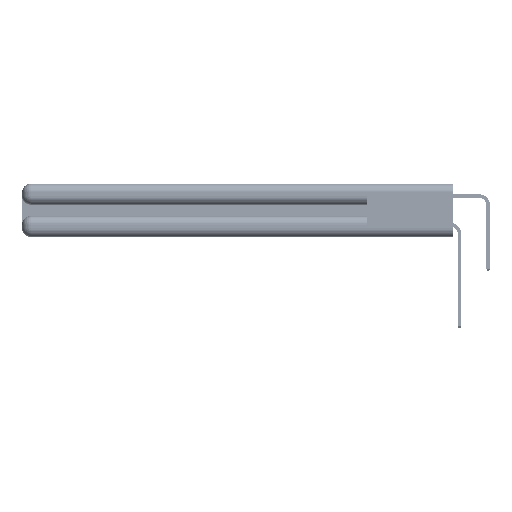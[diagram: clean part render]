
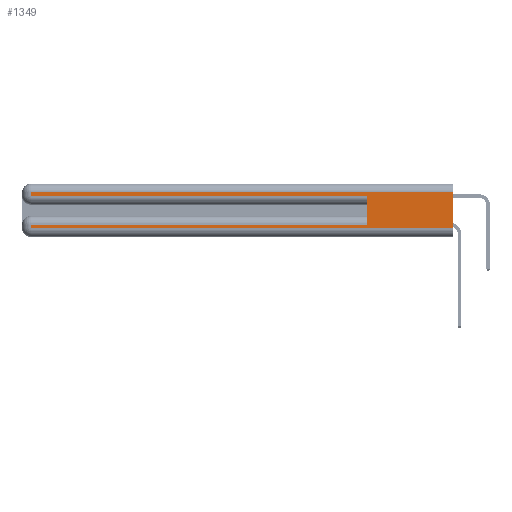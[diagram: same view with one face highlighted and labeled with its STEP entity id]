
A CAD part, left-side view. The second image highlights one B-rep face of the part: STEP entity #1349.
In plain terms, the highlighted planar face has unit normal (-1, 0, 0).
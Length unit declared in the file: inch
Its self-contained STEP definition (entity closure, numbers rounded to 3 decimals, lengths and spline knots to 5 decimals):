
#1305 = VERTEX_POINT ( 'NONE', #24181 ) ;
#1349 = ADVANCED_FACE ( 'NONE', ( #40857 ), #50335, .F. ) ;
#1712 = CARTESIAN_POINT ( 'NONE',  ( 0., 2.94, 0.37 ) ) ;
#1881 = DIRECTION ( 'NONE',  ( 0., 0., -1. ) ) ;
#2327 = ORIENTED_EDGE ( 'NONE', *, *, #28210, .T. ) ;
#2389 = CARTESIAN_POINT ( 'NONE',  ( 0., 0.6, 0.285 ) ) ;
#3100 = LINE ( 'NONE', #1712, #26706 ) ;
#3513 = ORIENTED_EDGE ( 'NONE', *, *, #25145, .F. ) ;
#4323 = VECTOR ( 'NONE', #38355, 39.37008 ) ;
#5999 = ORIENTED_EDGE ( 'NONE', *, *, #50599, .T. ) ;
#6085 = DIRECTION ( 'NONE',  ( 0., -1., 0. ) ) ;
#6158 = DIRECTION ( 'NONE',  ( 0., 0., -1. ) ) ;
#6929 = CARTESIAN_POINT ( 'NONE',  ( 0., 0., 0.37 ) ) ;
#7880 = VERTEX_POINT ( 'NONE', #20108 ) ;
#9024 = DIRECTION ( 'NONE',  ( 1., 0., 0. ) ) ;
#9645 = AXIS2_PLACEMENT_3D ( 'NONE', #6929, #9024, #1881 ) ;
#10930 = EDGE_CURVE ( 'NONE', #42783, #17025, #35552, .T. ) ;
#11955 = VECTOR ( 'NONE', #29552, 39.37008 ) ;
#14741 = LINE ( 'NONE', #33922, #4323 ) ;
#16319 = VERTEX_POINT ( 'NONE', #31454 ) ;
#17025 = VERTEX_POINT ( 'NONE', #48418 ) ;
#18938 = CARTESIAN_POINT ( 'NONE',  ( 0., 0., 0.06 ) ) ;
#20108 = CARTESIAN_POINT ( 'NONE',  ( 0., 0.6, 0.085 ) ) ;
#20200 = EDGE_LOOP ( 'NONE', ( #48483, #39694, #45628, #2327, #3513, #5999, #41041, #22214 ) ) ;
#22214 = ORIENTED_EDGE ( 'NONE', *, *, #25523, .T. ) ;
#23683 = EDGE_CURVE ( 'NONE', #1305, #43555, #26998, .T. ) ;
#24181 = CARTESIAN_POINT ( 'NONE',  ( 0., 0., 0.31 ) ) ;
#24269 = LINE ( 'NONE', #51905, #33285 ) ;
#25076 = CARTESIAN_POINT ( 'NONE',  ( 0., 2.94, 0.37 ) ) ;
#25145 = EDGE_CURVE ( 'NONE', #7880, #25656, #35852, .T. ) ;
#25523 = EDGE_CURVE ( 'NONE', #38308, #43555, #41304, .T. ) ;
#25656 = VERTEX_POINT ( 'NONE', #2389 ) ;
#25998 = CARTESIAN_POINT ( 'NONE',  ( 0., 0., 0.31 ) ) ;
#26706 = VECTOR ( 'NONE', #6158, 39.37008 ) ;
#26894 = EDGE_CURVE ( 'NONE', #16319, #38308, #3100, .T. ) ;
#26998 = LINE ( 'NONE', #37374, #38736 ) ;
#28210 = EDGE_CURVE ( 'NONE', #17025, #25656, #14741, .T. ) ;
#29552 = DIRECTION ( 'NONE',  ( 0., 0., -1. ) ) ;
#31454 = CARTESIAN_POINT ( 'NONE',  ( 0., 2.94, 0.085 ) ) ;
#33285 = VECTOR ( 'NONE', #38747, 39.37008 ) ;
#33922 = CARTESIAN_POINT ( 'NONE',  ( 0., 0., 0.285 ) ) ;
#34180 = VECTOR ( 'NONE', #56927, 39.37008 ) ;
#35552 = LINE ( 'NONE', #25076, #11955 ) ;
#35852 = LINE ( 'NONE', #47493, #46197 ) ;
#36824 = CARTESIAN_POINT ( 'NONE',  ( 0., 2.94, 0.31 ) ) ;
#37374 = CARTESIAN_POINT ( 'NONE',  ( 0., 0., 0.37 ) ) ;
#38308 = VERTEX_POINT ( 'NONE', #53498 ) ;
#38355 = DIRECTION ( 'NONE',  ( 0., -1., 0. ) ) ;
#38736 = VECTOR ( 'NONE', #41822, 39.37008 ) ;
#38747 = DIRECTION ( 'NONE',  ( 0., 1., 0. ) ) ;
#39694 = ORIENTED_EDGE ( 'NONE', *, *, #49041, .T. ) ;
#40857 = FACE_OUTER_BOUND ( 'NONE', #20200, .T. ) ;
#41041 = ORIENTED_EDGE ( 'NONE', *, *, #26894, .T. ) ;
#41304 = LINE ( 'NONE', #18938, #50284 ) ;
#41822 = DIRECTION ( 'NONE',  ( 0., 0., -1. ) ) ;
#42783 = VERTEX_POINT ( 'NONE', #36824 ) ;
#43555 = VERTEX_POINT ( 'NONE', #55727 ) ;
#45628 = ORIENTED_EDGE ( 'NONE', *, *, #10930, .T. ) ;
#46197 = VECTOR ( 'NONE', #51918, 39.37008 ) ;
#47493 = CARTESIAN_POINT ( 'NONE',  ( 0., 0.6, 0.145 ) ) ;
#48418 = CARTESIAN_POINT ( 'NONE',  ( 0., 2.94, 0.285 ) ) ;
#48483 = ORIENTED_EDGE ( 'NONE', *, *, #23683, .F. ) ;
#49041 = EDGE_CURVE ( 'NONE', #1305, #42783, #56307, .T. ) ;
#50284 = VECTOR ( 'NONE', #6085, 39.37008 ) ;
#50335 = PLANE ( 'NONE',  #9645 ) ;
#50599 = EDGE_CURVE ( 'NONE', #7880, #16319, #24269, .T. ) ;
#51905 = CARTESIAN_POINT ( 'NONE',  ( 0., 0., 0.085 ) ) ;
#51918 = DIRECTION ( 'NONE',  ( 0., 0., 1. ) ) ;
#53498 = CARTESIAN_POINT ( 'NONE',  ( 0., 2.94, 0.06 ) ) ;
#55727 = CARTESIAN_POINT ( 'NONE',  ( 0., 0., 0.06 ) ) ;
#56307 = LINE ( 'NONE', #25998, #34180 ) ;
#56927 = DIRECTION ( 'NONE',  ( 0., 1., 0. ) ) ;
